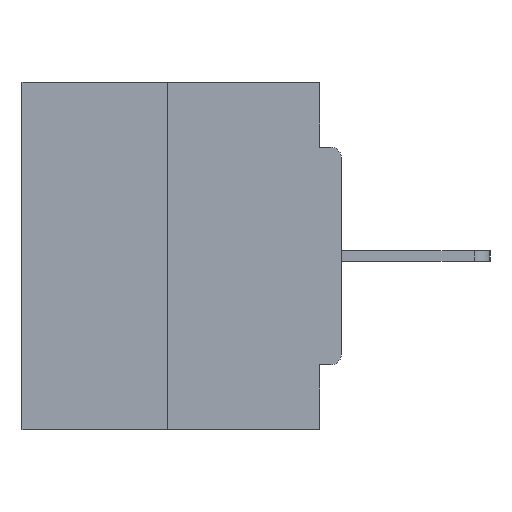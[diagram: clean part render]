
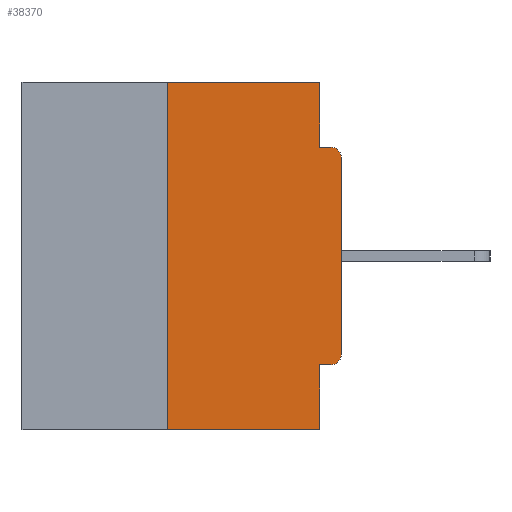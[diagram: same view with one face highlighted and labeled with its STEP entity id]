
A CAD part, left-side view. The second image highlights one B-rep face of the part: STEP entity #38370.
In plain terms, the highlighted planar face has unit normal (-1, 0, 0).
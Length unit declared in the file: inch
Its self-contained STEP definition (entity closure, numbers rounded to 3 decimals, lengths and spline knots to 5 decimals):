
#452 = ORIENTED_EDGE ( 'NONE', *, *, #36312, .T. ) ;
#3065 = CARTESIAN_POINT ( 'NONE',  ( 0., 0., -0.1085 ) ) ;
#3193 = LINE ( 'NONE', #15152, #14496 ) ;
#3218 = LINE ( 'NONE', #38311, #6745 ) ;
#3803 = CARTESIAN_POINT ( 'NONE',  ( 0., 0.25, -0.5 ) ) ;
#4534 = EDGE_CURVE ( 'NONE', #27913, #19149, #14602, .T. ) ;
#4673 = ORIENTED_EDGE ( 'NONE', *, *, #10199, .T. ) ;
#5181 = VECTOR ( 'NONE', #27586, 39.37008 ) ;
#5628 = ORIENTED_EDGE ( 'NONE', *, *, #38195, .F. ) ;
#5735 = DIRECTION ( 'NONE',  ( 0., 0., -1. ) ) ;
#5862 = DIRECTION ( 'NONE',  ( -1., 0., 0. ) ) ;
#6103 = CARTESIAN_POINT ( 'NONE',  ( 0., 0.46, -0.5 ) ) ;
#6196 = LINE ( 'NONE', #23873, #5181 ) ;
#6201 = EDGE_CURVE ( 'NONE', #29114, #19411, #35732, .T. ) ;
#6283 = AXIS2_PLACEMENT_3D ( 'NONE', #8429, #5862, #32943 ) ;
#6745 = VECTOR ( 'NONE', #27148, 39.37008 ) ;
#6991 = CARTESIAN_POINT ( 'NONE',  ( 0., 0.25, 0. ) ) ;
#8429 = CARTESIAN_POINT ( 'NONE',  ( 0., 0.015, -0.1085 ) ) ;
#9466 = VECTOR ( 'NONE', #25377, 39.37008 ) ;
#9531 = ORIENTED_EDGE ( 'NONE', *, *, #4534, .T. ) ;
#9761 = LINE ( 'NONE', #6991, #11630 ) ;
#10199 = EDGE_CURVE ( 'NONE', #19149, #35019, #6196, .T. ) ;
#10567 = VERTEX_POINT ( 'NONE', #18885 ) ;
#10683 = VECTOR ( 'NONE', #33290, 39.37008 ) ;
#11416 = CARTESIAN_POINT ( 'NONE',  ( 0., 0.031, 0. ) ) ;
#11630 = VECTOR ( 'NONE', #12876, 39.37008 ) ;
#12192 = EDGE_CURVE ( 'NONE', #16120, #29114, #3218, .T. ) ;
#12876 = DIRECTION ( 'NONE',  ( 0., 0., 1. ) ) ;
#14409 = CARTESIAN_POINT ( 'NONE',  ( 0., 0.015, -0.0935 ) ) ;
#14496 = VECTOR ( 'NONE', #5735, 39.37008 ) ;
#14602 = CIRCLE ( 'NONE', #32133, 0.015 ) ;
#15030 = CARTESIAN_POINT ( 'NONE',  ( 0., 0.015, -0.4065 ) ) ;
#15152 = CARTESIAN_POINT ( 'NONE',  ( 0., 0.031, -0.5 ) ) ;
#15344 = VERTEX_POINT ( 'NONE', #14409 ) ;
#15378 = VERTEX_POINT ( 'NONE', #3803 ) ;
#16120 = VERTEX_POINT ( 'NONE', #35308 ) ;
#18076 = DIRECTION ( 'NONE',  ( 0., -1., 0. ) ) ;
#18178 = CARTESIAN_POINT ( 'NONE',  ( 0., 0.031, 0. ) ) ;
#18885 = CARTESIAN_POINT ( 'NONE',  ( 0., 0.031, -0.4065 ) ) ;
#19149 = VERTEX_POINT ( 'NONE', #27118 ) ;
#19411 = VERTEX_POINT ( 'NONE', #25523 ) ;
#19493 = CARTESIAN_POINT ( 'NONE',  ( 0., 0., -0.0935 ) ) ;
#20031 = DIRECTION ( 'NONE',  ( 0., 0., -1. ) ) ;
#20094 = CARTESIAN_POINT ( 'NONE',  ( 0., 0.015, -0.3915 ) ) ;
#20583 = VECTOR ( 'NONE', #29451, 39.37008 ) ;
#21314 = CARTESIAN_POINT ( 'NONE',  ( 0., 0., -0.4065 ) ) ;
#21323 = CIRCLE ( 'NONE', #6283, 0.015 ) ;
#22656 = DIRECTION ( 'NONE',  ( -1., 0., 0. ) ) ;
#23380 = EDGE_CURVE ( 'NONE', #10567, #26686, #3193, .T. ) ;
#23873 = CARTESIAN_POINT ( 'NONE',  ( 0., 0., 0. ) ) ;
#24256 = LINE ( 'NONE', #21314, #10683 ) ;
#25339 = EDGE_LOOP ( 'NONE', ( #30348, #35373, #25783, #25533, #5628, #9531, #4673, #452, #32109, #34805 ) ) ;
#25377 = DIRECTION ( 'NONE',  ( 0., -1., 0. ) ) ;
#25523 = CARTESIAN_POINT ( 'NONE',  ( 0., 0.031, -0.0935 ) ) ;
#25533 = ORIENTED_EDGE ( 'NONE', *, *, #23380, .F. ) ;
#25755 = VECTOR ( 'NONE', #18076, 39.37008 ) ;
#25783 = ORIENTED_EDGE ( 'NONE', *, *, #37269, .T. ) ;
#25924 = PLANE ( 'NONE',  #38240 ) ;
#26686 = VERTEX_POINT ( 'NONE', #30311 ) ;
#27118 = CARTESIAN_POINT ( 'NONE',  ( 0., 0., -0.3915 ) ) ;
#27148 = DIRECTION ( 'NONE',  ( 0., -1., 0. ) ) ;
#27586 = DIRECTION ( 'NONE',  ( 0., 0., 1. ) ) ;
#27913 = VERTEX_POINT ( 'NONE', #15030 ) ;
#28921 = DIRECTION ( 'NONE',  ( 0., 0., -1. ) ) ;
#29114 = VERTEX_POINT ( 'NONE', #18178 ) ;
#29206 = EDGE_CURVE ( 'NONE', #15378, #16120, #9761, .T. ) ;
#29451 = DIRECTION ( 'NONE',  ( 0., 0., -1. ) ) ;
#30311 = CARTESIAN_POINT ( 'NONE',  ( 0., 0.031, -0.5 ) ) ;
#30348 = ORIENTED_EDGE ( 'NONE', *, *, #12192, .F. ) ;
#31437 = LINE ( 'NONE', #19493, #9466 ) ;
#32109 = ORIENTED_EDGE ( 'NONE', *, *, #36824, .F. ) ;
#32133 = AXIS2_PLACEMENT_3D ( 'NONE', #20094, #22656, #28921 ) ;
#32943 = DIRECTION ( 'NONE',  ( 0., 0., -1. ) ) ;
#32992 = LINE ( 'NONE', #6103, #25755 ) ;
#33290 = DIRECTION ( 'NONE',  ( 0., 1., 0. ) ) ;
#34755 = CARTESIAN_POINT ( 'NONE',  ( 0., 0.46, 0. ) ) ;
#34805 = ORIENTED_EDGE ( 'NONE', *, *, #6201, .F. ) ;
#35019 = VERTEX_POINT ( 'NONE', #3065 ) ;
#35133 = FACE_OUTER_BOUND ( 'NONE', #25339, .T. ) ;
#35308 = CARTESIAN_POINT ( 'NONE',  ( 0., 0.25, 0. ) ) ;
#35373 = ORIENTED_EDGE ( 'NONE', *, *, #29206, .F. ) ;
#35732 = LINE ( 'NONE', #11416, #20583 ) ;
#36312 = EDGE_CURVE ( 'NONE', #35019, #15344, #21323, .T. ) ;
#36824 = EDGE_CURVE ( 'NONE', #19411, #15344, #31437, .T. ) ;
#37269 = EDGE_CURVE ( 'NONE', #15378, #26686, #32992, .T. ) ;
#37875 = DIRECTION ( 'NONE',  ( 1., 0., 0. ) ) ;
#38195 = EDGE_CURVE ( 'NONE', #27913, #10567, #24256, .T. ) ;
#38240 = AXIS2_PLACEMENT_3D ( 'NONE', #34755, #37875, #20031 ) ;
#38311 = CARTESIAN_POINT ( 'NONE',  ( 0., 0.46, 0. ) ) ;
#38370 = ADVANCED_FACE ( 'NONE', ( #35133 ), #25924, .F. ) ;
